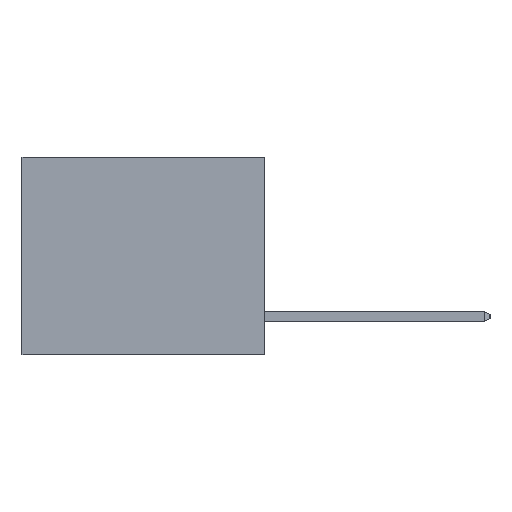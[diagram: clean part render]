
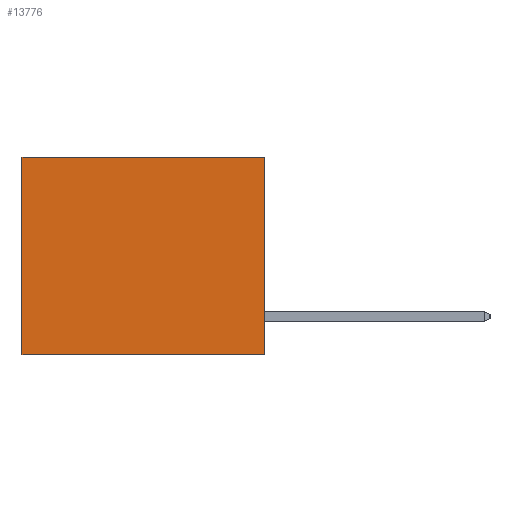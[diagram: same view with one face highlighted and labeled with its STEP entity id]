
A CAD part, left-side view. The second image highlights one B-rep face of the part: STEP entity #13776.
In plain terms, the highlighted planar face has unit normal (-1, 0, 0).
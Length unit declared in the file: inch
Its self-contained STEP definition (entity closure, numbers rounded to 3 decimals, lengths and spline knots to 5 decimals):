
#1566 = VERTEX_POINT ( 'NONE', #22543 ) ;
#1738 = LINE ( 'NONE', #14776, #23999 ) ;
#2059 = PLANE ( 'NONE',  #2849 ) ;
#2362 = EDGE_CURVE ( 'NONE', #21700, #1566, #8232, .T. ) ;
#2849 = AXIS2_PLACEMENT_3D ( 'NONE', #27144, #6734, #8853 ) ;
#3383 = ORIENTED_EDGE ( 'NONE', *, *, #2362, .F. ) ;
#3717 = VECTOR ( 'NONE', #17010, 39.37008 ) ;
#4399 = VECTOR ( 'NONE', #5813, 39.37008 ) ;
#5813 = DIRECTION ( 'NONE',  ( 0., 0., -1. ) ) ;
#6734 = DIRECTION ( 'NONE',  ( 1., 0., 0. ) ) ;
#8024 = LINE ( 'NONE', #14707, #3717 ) ;
#8232 = LINE ( 'NONE', #10290, #27600 ) ;
#8417 = EDGE_LOOP ( 'NONE', ( #27734, #3383, #13353, #14168 ) ) ;
#8588 = EDGE_CURVE ( 'NONE', #27081, #21700, #1738, .T. ) ;
#8853 = DIRECTION ( 'NONE',  ( 0., 0., -1. ) ) ;
#9679 = CARTESIAN_POINT ( 'NONE',  ( 0.3165, 0., 0. ) ) ;
#10290 = CARTESIAN_POINT ( 'NONE',  ( 0.3165, 0., -0.49 ) ) ;
#10397 = FACE_OUTER_BOUND ( 'NONE', #8417, .T. ) ;
#12177 = VERTEX_POINT ( 'NONE', #21685 ) ;
#12733 = DIRECTION ( 'NONE',  ( 0., 0., -1. ) ) ;
#13353 = ORIENTED_EDGE ( 'NONE', *, *, #8588, .F. ) ;
#13776 = ADVANCED_FACE ( 'NONE', ( #10397 ), #2059, .F. ) ;
#14168 = ORIENTED_EDGE ( 'NONE', *, *, #16259, .T. ) ;
#14707 = CARTESIAN_POINT ( 'NONE',  ( 0.3165, 0., 0. ) ) ;
#14776 = CARTESIAN_POINT ( 'NONE',  ( 0.3165, 0., -0.49 ) ) ;
#16259 = EDGE_CURVE ( 'NONE', #27081, #12177, #8024, .T. ) ;
#17010 = DIRECTION ( 'NONE',  ( 0., 1., 0. ) ) ;
#19443 = DIRECTION ( 'NONE',  ( 0., 1., 0. ) ) ;
#21685 = CARTESIAN_POINT ( 'NONE',  ( 0.3165, 0.6, 0. ) ) ;
#21700 = VERTEX_POINT ( 'NONE', #25109 ) ;
#22543 = CARTESIAN_POINT ( 'NONE',  ( 0.3165, 0.6, -0.49 ) ) ;
#23793 = LINE ( 'NONE', #26377, #4399 ) ;
#23999 = VECTOR ( 'NONE', #12733, 39.37008 ) ;
#25109 = CARTESIAN_POINT ( 'NONE',  ( 0.3165, 0., -0.49 ) ) ;
#26377 = CARTESIAN_POINT ( 'NONE',  ( 0.3165, 0.6, -0.49 ) ) ;
#27081 = VERTEX_POINT ( 'NONE', #9679 ) ;
#27144 = CARTESIAN_POINT ( 'NONE',  ( 0.3165, 0., -0.49 ) ) ;
#27600 = VECTOR ( 'NONE', #19443, 39.37008 ) ;
#27734 = ORIENTED_EDGE ( 'NONE', *, *, #28417, .T. ) ;
#28417 = EDGE_CURVE ( 'NONE', #12177, #1566, #23793, .T. ) ;
